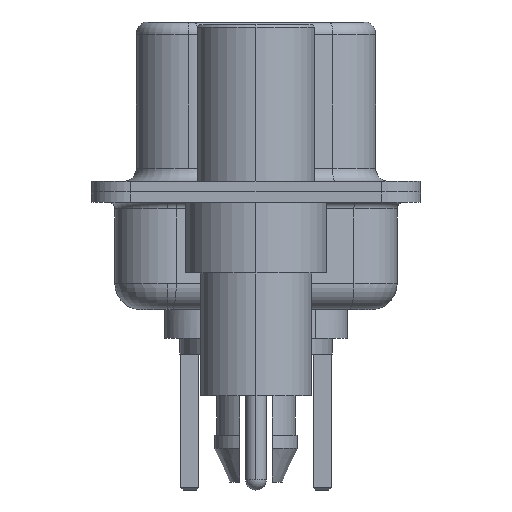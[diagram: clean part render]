
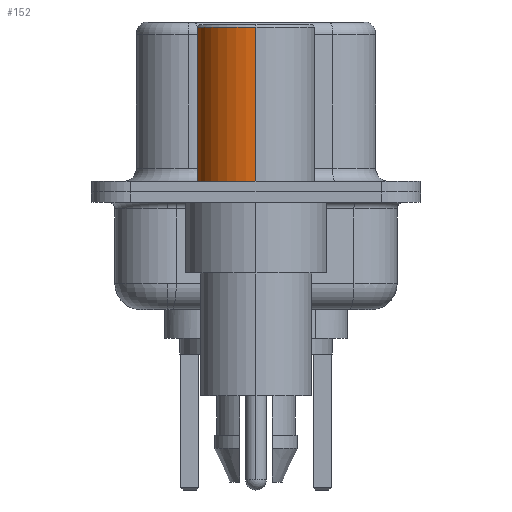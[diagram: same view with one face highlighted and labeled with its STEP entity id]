
A CAD part, left-side view. The second image highlights one B-rep face of the part: STEP entity #152.
In plain terms, the highlighted cylindrical face has radius 2.25 mm (diameter 4.5 mm), a partial arc.
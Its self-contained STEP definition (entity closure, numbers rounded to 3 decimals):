
#90 = ORIENTED_EDGE ( 'NONE', *, *, #16828, .T. ) ;
#152 = ADVANCED_FACE ( 'NONE', ( #2425 ), #10282, .T. ) ;
#1083 = AXIS2_PLACEMENT_3D ( 'NONE', #2144, #13226, #3714 ) ;
#1331 = CARTESIAN_POINT ( 'NONE',  ( -2.25, 0., 0.581 ) ) ;
#2144 = CARTESIAN_POINT ( 'NONE',  ( 0., 0., 6.3 ) ) ;
#2425 = FACE_OUTER_BOUND ( 'NONE', #18103, .T. ) ;
#3113 = EDGE_CURVE ( 'NONE', #15295, #9855, #20386, .T. ) ;
#3182 = CARTESIAN_POINT ( 'NONE',  ( 2.25, 0., 0.4 ) ) ;
#3714 = DIRECTION ( 'NONE',  ( 1., 0., 0. ) ) ;
#4280 = CARTESIAN_POINT ( 'NONE',  ( -2.25, 0., 0.4 ) ) ;
#5088 = DIRECTION ( 'NONE',  ( 0., 0., 1. ) ) ;
#5174 = LINE ( 'NONE', #1331, #19483 ) ;
#5299 = CARTESIAN_POINT ( 'NONE',  ( 0., 0., 0.4 ) ) ;
#5503 = DIRECTION ( 'NONE',  ( 1., 0., 0. ) ) ;
#6275 = EDGE_CURVE ( 'NONE', #15101, #15301, #5174, .T. ) ;
#6877 = DIRECTION ( 'NONE',  ( 1., 0., 0. ) ) ;
#7736 = CARTESIAN_POINT ( 'NONE',  ( 2.25, 0., 6.3 ) ) ;
#8089 = ORIENTED_EDGE ( 'NONE', *, *, #6275, .T. ) ;
#9855 = VERTEX_POINT ( 'NONE', #7736 ) ;
#10282 = CYLINDRICAL_SURFACE ( 'NONE', #18616, 2.25 ) ;
#11625 = CIRCLE ( 'NONE', #18998, 2.25 ) ;
#12754 = CARTESIAN_POINT ( 'NONE',  ( 0., 0., 0.581 ) ) ;
#13226 = DIRECTION ( 'NONE',  ( 0., 0., 1. ) ) ;
#14023 = DIRECTION ( 'NONE',  ( 0., 0., 1. ) ) ;
#15101 = VERTEX_POINT ( 'NONE', #4280 ) ;
#15295 = VERTEX_POINT ( 'NONE', #3182 ) ;
#15301 = VERTEX_POINT ( 'NONE', #15816 ) ;
#15816 = CARTESIAN_POINT ( 'NONE',  ( -2.25, 0., 6.3 ) ) ;
#16036 = ORIENTED_EDGE ( 'NONE', *, *, #18949, .F. ) ;
#16155 = CARTESIAN_POINT ( 'NONE',  ( 2.25, 0., 0.581 ) ) ;
#16332 = DIRECTION ( 'NONE',  ( 0., 0., 1. ) ) ;
#16610 = VECTOR ( 'NONE', #14023, 1000. ) ;
#16828 = EDGE_CURVE ( 'NONE', #15295, #15101, #11625, .T. ) ;
#16931 = DIRECTION ( 'NONE',  ( 0., 0., 1. ) ) ;
#18103 = EDGE_LOOP ( 'NONE', ( #90, #8089, #16036, #20189 ) ) ;
#18616 = AXIS2_PLACEMENT_3D ( 'NONE', #12754, #16931, #5503 ) ;
#18949 = EDGE_CURVE ( 'NONE', #9855, #15301, #19945, .T. ) ;
#18998 = AXIS2_PLACEMENT_3D ( 'NONE', #5299, #16332, #6877 ) ;
#19483 = VECTOR ( 'NONE', #5088, 1000. ) ;
#19945 = CIRCLE ( 'NONE', #1083, 2.25 ) ;
#20189 = ORIENTED_EDGE ( 'NONE', *, *, #3113, .F. ) ;
#20386 = LINE ( 'NONE', #16155, #16610 ) ;
